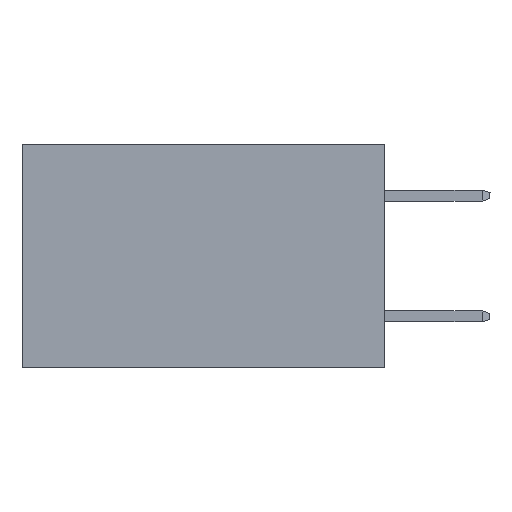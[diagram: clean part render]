
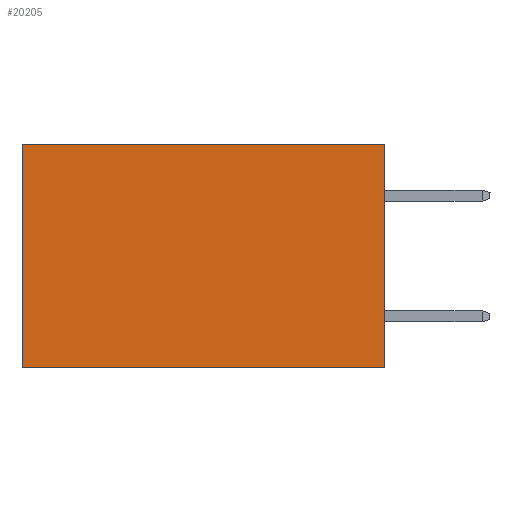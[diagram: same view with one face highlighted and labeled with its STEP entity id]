
A CAD part, left-side view. The second image highlights one B-rep face of the part: STEP entity #20205.
In plain terms, the highlighted planar face has unit normal (-1, 0, 0).
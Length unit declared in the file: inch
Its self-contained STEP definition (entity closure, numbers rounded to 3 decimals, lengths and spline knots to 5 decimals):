
#45 = DIRECTION ( 'NONE',  ( 0., 1., 0. ) ) ;
#1065 = CARTESIAN_POINT ( 'NONE',  ( 0.298, 0., -0.37 ) ) ;
#4199 = FACE_OUTER_BOUND ( 'NONE', #18911, .T. ) ;
#4291 = CARTESIAN_POINT ( 'NONE',  ( 0.298, 0., 0. ) ) ;
#4380 = ORIENTED_EDGE ( 'NONE', *, *, #21810, .F. ) ;
#4913 = ORIENTED_EDGE ( 'NONE', *, *, #11022, .F. ) ;
#6032 = CARTESIAN_POINT ( 'NONE',  ( 0.298, 0., 0. ) ) ;
#6460 = CARTESIAN_POINT ( 'NONE',  ( 0.298, 0., 0. ) ) ;
#7484 = ORIENTED_EDGE ( 'NONE', *, *, #7711, .T. ) ;
#7649 = CARTESIAN_POINT ( 'NONE',  ( 0.298, 0.6, 0. ) ) ;
#7711 = EDGE_CURVE ( 'NONE', #12792, #11080, #14751, .T. ) ;
#8368 = VECTOR ( 'NONE', #20696, 39.37008 ) ;
#9699 = DIRECTION ( 'NONE',  ( 0., 0., -1. ) ) ;
#9994 = VECTOR ( 'NONE', #45, 39.37008 ) ;
#10053 = PLANE ( 'NONE',  #12251 ) ;
#10613 = LINE ( 'NONE', #6460, #8368 ) ;
#10652 = CARTESIAN_POINT ( 'NONE',  ( 0.298, 0.6, 0. ) ) ;
#11022 = EDGE_CURVE ( 'NONE', #21153, #17635, #19970, .T. ) ;
#11080 = VERTEX_POINT ( 'NONE', #10652 ) ;
#11968 = DIRECTION ( 'NONE',  ( 1., 0., 0. ) ) ;
#12251 = AXIS2_PLACEMENT_3D ( 'NONE', #6032, #11968, #22407 ) ;
#12750 = EDGE_CURVE ( 'NONE', #11080, #17635, #14478, .T. ) ;
#12792 = VERTEX_POINT ( 'NONE', #15972 ) ;
#14478 = LINE ( 'NONE', #7649, #22718 ) ;
#14751 = LINE ( 'NONE', #4291, #17596 ) ;
#15293 = ORIENTED_EDGE ( 'NONE', *, *, #12750, .T. ) ;
#15972 = CARTESIAN_POINT ( 'NONE',  ( 0.298, 0., 0. ) ) ;
#17596 = VECTOR ( 'NONE', #18400, 39.37008 ) ;
#17635 = VERTEX_POINT ( 'NONE', #19912 ) ;
#18400 = DIRECTION ( 'NONE',  ( 0., 1., 0. ) ) ;
#18911 = EDGE_LOOP ( 'NONE', ( #15293, #4913, #4380, #7484 ) ) ;
#19912 = CARTESIAN_POINT ( 'NONE',  ( 0.298, 0.6, -0.37 ) ) ;
#19970 = LINE ( 'NONE', #24712, #9994 ) ;
#20205 = ADVANCED_FACE ( 'NONE', ( #4199 ), #10053, .F. ) ;
#20696 = DIRECTION ( 'NONE',  ( 0., 0., -1. ) ) ;
#21153 = VERTEX_POINT ( 'NONE', #1065 ) ;
#21810 = EDGE_CURVE ( 'NONE', #12792, #21153, #10613, .T. ) ;
#22407 = DIRECTION ( 'NONE',  ( 0., 0., -1. ) ) ;
#22718 = VECTOR ( 'NONE', #9699, 39.37008 ) ;
#24712 = CARTESIAN_POINT ( 'NONE',  ( 0.298, 0., -0.37 ) ) ;
